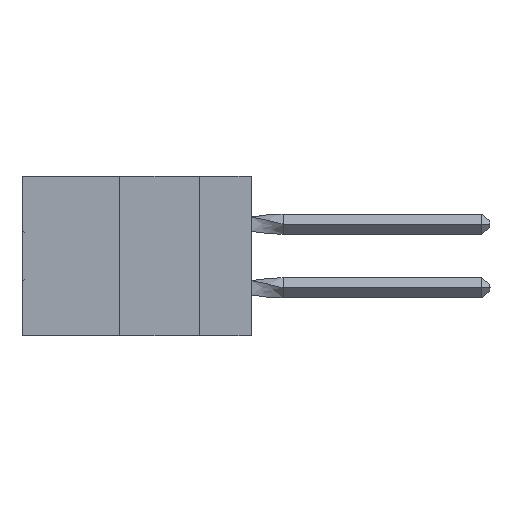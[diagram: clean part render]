
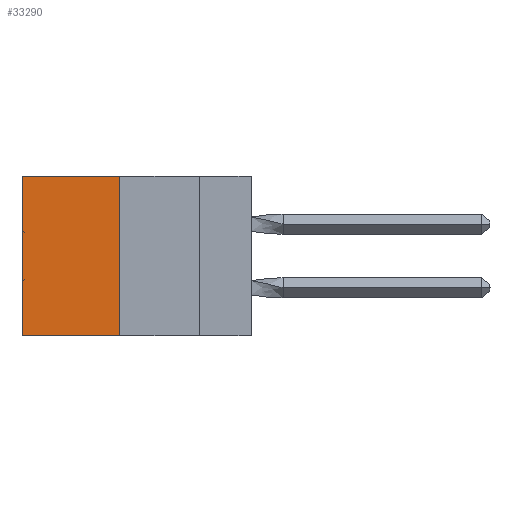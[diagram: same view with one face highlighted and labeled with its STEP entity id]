
A CAD part, left-side view. The second image highlights one B-rep face of the part: STEP entity #33290.
In plain terms, the highlighted planar face has unit normal (-1, 0, 0).
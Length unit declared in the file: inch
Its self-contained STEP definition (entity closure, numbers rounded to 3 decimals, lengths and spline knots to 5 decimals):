
#1408 = DIRECTION ( 'NONE',  ( 0., 0., -1. ) ) ;
#1982 = CARTESIAN_POINT ( 'NONE',  ( 0.305, 0.72, -0.5 ) ) ;
#2088 = VECTOR ( 'NONE', #49929, 39.37008 ) ;
#2679 = FACE_OUTER_BOUND ( 'NONE', #2930, .T. ) ;
#2930 = EDGE_LOOP ( 'NONE', ( #5074, #15619, #48248, #21800 ) ) ;
#3842 = EDGE_CURVE ( 'NONE', #4750, #32372, #30779, .T. ) ;
#4094 = CARTESIAN_POINT ( 'NONE',  ( 0.305, 0.413, -0.5 ) ) ;
#4750 = VERTEX_POINT ( 'NONE', #39962 ) ;
#5074 = ORIENTED_EDGE ( 'NONE', *, *, #9195, .T. ) ;
#7541 = DIRECTION ( 'NONE',  ( 1., 0., 0. ) ) ;
#9195 = EDGE_CURVE ( 'NONE', #32372, #11555, #21022, .T. ) ;
#11555 = VERTEX_POINT ( 'NONE', #30316 ) ;
#12120 = LINE ( 'NONE', #44044, #15348 ) ;
#14444 = VECTOR ( 'NONE', #51627, 39.37008 ) ;
#15348 = VECTOR ( 'NONE', #18988, 39.37008 ) ;
#15619 = ORIENTED_EDGE ( 'NONE', *, *, #38983, .F. ) ;
#18988 = DIRECTION ( 'NONE',  ( 0., 1., 0. ) ) ;
#21022 = LINE ( 'NONE', #1982, #14444 ) ;
#21800 = ORIENTED_EDGE ( 'NONE', *, *, #3842, .T. ) ;
#22589 = CARTESIAN_POINT ( 'NONE',  ( 0.305, 0.413, -0.5 ) ) ;
#29089 = PLANE ( 'NONE',  #31966 ) ;
#30316 = CARTESIAN_POINT ( 'NONE',  ( 0.305, 0.72, -0.5 ) ) ;
#30779 = LINE ( 'NONE', #54057, #2088 ) ;
#31966 = AXIS2_PLACEMENT_3D ( 'NONE', #4094, #7541, #53491 ) ;
#32073 = VECTOR ( 'NONE', #1408, 39.37008 ) ;
#32372 = VERTEX_POINT ( 'NONE', #42761 ) ;
#33290 = ADVANCED_FACE ( 'NONE', ( #2679 ), #29089, .F. ) ;
#38983 = EDGE_CURVE ( 'NONE', #47715, #11555, #12120, .T. ) ;
#39962 = CARTESIAN_POINT ( 'NONE',  ( 0.305, 0.413, 0. ) ) ;
#42761 = CARTESIAN_POINT ( 'NONE',  ( 0.305, 0.72, 0. ) ) ;
#44044 = CARTESIAN_POINT ( 'NONE',  ( 0.305, 0.413, -0.5 ) ) ;
#47715 = VERTEX_POINT ( 'NONE', #22589 ) ;
#48248 = ORIENTED_EDGE ( 'NONE', *, *, #50110, .F. ) ;
#49929 = DIRECTION ( 'NONE',  ( 0., 1., 0. ) ) ;
#50110 = EDGE_CURVE ( 'NONE', #4750, #47715, #51746, .T. ) ;
#51627 = DIRECTION ( 'NONE',  ( 0., 0., -1. ) ) ;
#51746 = LINE ( 'NONE', #52828, #32073 ) ;
#52828 = CARTESIAN_POINT ( 'NONE',  ( 0.305, 0.413, -0.5 ) ) ;
#53491 = DIRECTION ( 'NONE',  ( 0., 0., -1. ) ) ;
#54057 = CARTESIAN_POINT ( 'NONE',  ( 0.305, 0.413, 0. ) ) ;
